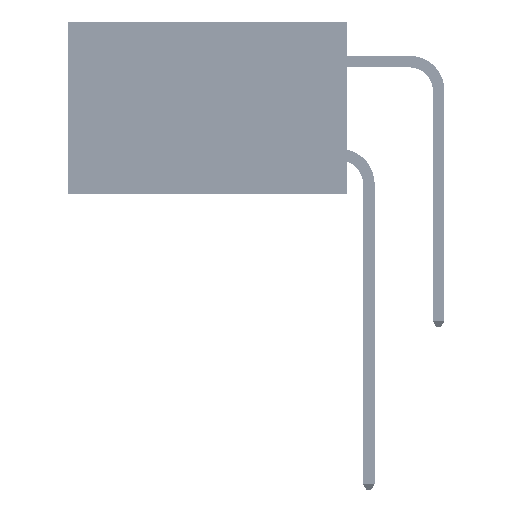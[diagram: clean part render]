
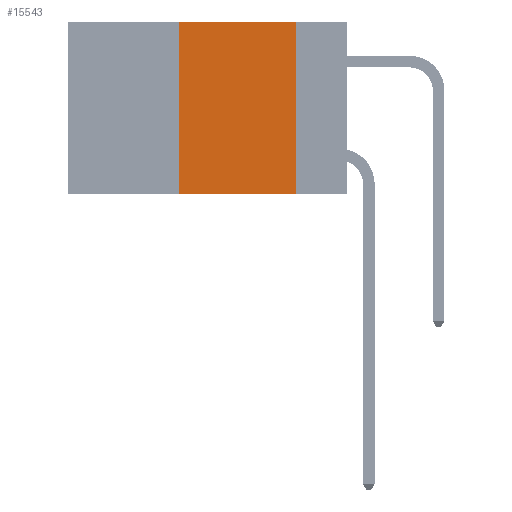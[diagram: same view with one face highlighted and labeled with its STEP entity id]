
A CAD part, left-side view. The second image highlights one B-rep face of the part: STEP entity #15543.
In plain terms, the highlighted planar face has unit normal (-1, 0, 0).
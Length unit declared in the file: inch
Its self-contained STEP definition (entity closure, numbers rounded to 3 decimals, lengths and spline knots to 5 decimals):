
#407 = DIRECTION ( 'NONE',  ( 0., -1., 0. ) ) ;
#1995 = CARTESIAN_POINT ( 'NONE',  ( 0., 0.11, 0. ) ) ;
#5550 = EDGE_LOOP ( 'NONE', ( #6083, #28435, #44804, #44465 ) ) ;
#5807 = VECTOR ( 'NONE', #7087, 39.37008 ) ;
#5978 = VERTEX_POINT ( 'NONE', #35573 ) ;
#6083 = ORIENTED_EDGE ( 'NONE', *, *, #30802, .F. ) ;
#7087 = DIRECTION ( 'NONE',  ( 0., 0., 1. ) ) ;
#8298 = VERTEX_POINT ( 'NONE', #19596 ) ;
#9590 = LINE ( 'NONE', #1995, #19132 ) ;
#11183 = EDGE_CURVE ( 'NONE', #25383, #21405, #31721, .T. ) ;
#12542 = LINE ( 'NONE', #39884, #5807 ) ;
#15543 = ADVANCED_FACE ( 'NONE', ( #29777 ), #45231, .F. ) ;
#16288 = CARTESIAN_POINT ( 'NONE',  ( 0., 0.11, -0.37 ) ) ;
#17643 = VECTOR ( 'NONE', #41040, 39.37008 ) ;
#18287 = VECTOR ( 'NONE', #407, 39.37008 ) ;
#19132 = VECTOR ( 'NONE', #44967, 39.37008 ) ;
#19596 = CARTESIAN_POINT ( 'NONE',  ( 0., 0.36, 0. ) ) ;
#20485 = AXIS2_PLACEMENT_3D ( 'NONE', #27060, #34281, #41505 ) ;
#21405 = VERTEX_POINT ( 'NONE', #16288 ) ;
#25383 = VERTEX_POINT ( 'NONE', #28560 ) ;
#27060 = CARTESIAN_POINT ( 'NONE',  ( 0., 0.6, 0. ) ) ;
#28435 = ORIENTED_EDGE ( 'NONE', *, *, #43985, .F. ) ;
#28560 = CARTESIAN_POINT ( 'NONE',  ( 0., 0.36, -0.37 ) ) ;
#29777 = FACE_OUTER_BOUND ( 'NONE', #5550, .T. ) ;
#30802 = EDGE_CURVE ( 'NONE', #5978, #21405, #9590, .T. ) ;
#31721 = LINE ( 'NONE', #44457, #17643 ) ;
#34281 = DIRECTION ( 'NONE',  ( 1., 0., 0. ) ) ;
#35573 = CARTESIAN_POINT ( 'NONE',  ( 0., 0.11, 0. ) ) ;
#39331 = EDGE_CURVE ( 'NONE', #25383, #8298, #12542, .T. ) ;
#39692 = LINE ( 'NONE', #39988, #18287 ) ;
#39884 = CARTESIAN_POINT ( 'NONE',  ( 0., 0.36, 0. ) ) ;
#39988 = CARTESIAN_POINT ( 'NONE',  ( 0., 0.6, 0. ) ) ;
#41040 = DIRECTION ( 'NONE',  ( 0., -1., 0. ) ) ;
#41505 = DIRECTION ( 'NONE',  ( 0., 0., -1. ) ) ;
#43985 = EDGE_CURVE ( 'NONE', #8298, #5978, #39692, .T. ) ;
#44457 = CARTESIAN_POINT ( 'NONE',  ( 0., 0.6, -0.37 ) ) ;
#44465 = ORIENTED_EDGE ( 'NONE', *, *, #11183, .T. ) ;
#44804 = ORIENTED_EDGE ( 'NONE', *, *, #39331, .F. ) ;
#44967 = DIRECTION ( 'NONE',  ( 0., 0., -1. ) ) ;
#45231 = PLANE ( 'NONE',  #20485 ) ;
